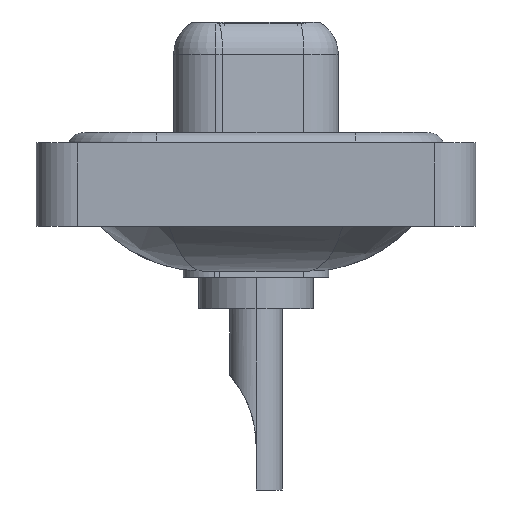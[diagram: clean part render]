
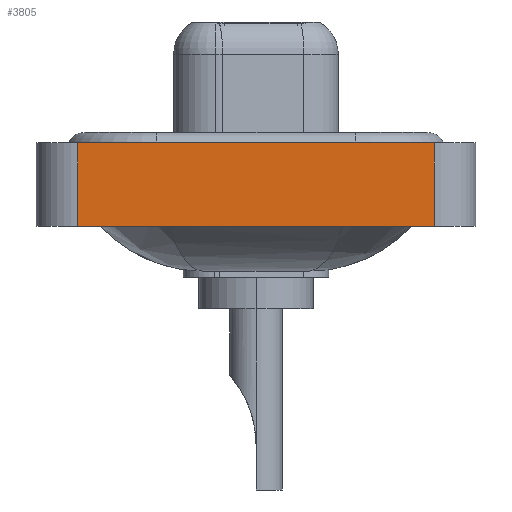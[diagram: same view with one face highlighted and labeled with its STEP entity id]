
A CAD part, left-side view. The second image highlights one B-rep face of the part: STEP entity #3805.
In plain terms, the highlighted planar face has unit normal (-1, 0, 0).
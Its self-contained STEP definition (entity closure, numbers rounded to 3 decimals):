
#897 = ORIENTED_EDGE ( 'NONE', *, *, #14200, .T. ) ;
#1288 = CARTESIAN_POINT ( 'NONE',  ( -7.25, -8.55, -3.6 ) ) ;
#1683 = PLANE ( 'NONE',  #7517 ) ;
#2058 = VECTOR ( 'NONE', #10575, 1000. ) ;
#2520 = CARTESIAN_POINT ( 'NONE',  ( -7.25, -8.55, -3.6 ) ) ;
#2913 = FACE_OUTER_BOUND ( 'NONE', #6104, .T. ) ;
#2992 = DIRECTION ( 'NONE',  ( 0., 0., 1. ) ) ;
#3805 = ADVANCED_FACE ( 'NONE', ( #2913 ), #1683, .T. ) ;
#3864 = EDGE_CURVE ( 'NONE', #12638, #15703, #9419, .T. ) ;
#4318 = ORIENTED_EDGE ( 'NONE', *, *, #7551, .F. ) ;
#4462 = CARTESIAN_POINT ( 'NONE',  ( -7.25, -8.55, -3.6 ) ) ;
#4849 = VECTOR ( 'NONE', #16111, 1000. ) ;
#5597 = DIRECTION ( 'NONE',  ( -1., 0., 0. ) ) ;
#5711 = ORIENTED_EDGE ( 'NONE', *, *, #15212, .F. ) ;
#6010 = CARTESIAN_POINT ( 'NONE',  ( -7.25, 8.55, -3.6 ) ) ;
#6104 = EDGE_LOOP ( 'NONE', ( #14749, #5711, #4318, #897 ) ) ;
#6641 = LINE ( 'NONE', #10410, #11677 ) ;
#7107 = DIRECTION ( 'NONE',  ( 0., -1., 0. ) ) ;
#7247 = VERTEX_POINT ( 'NONE', #6010 ) ;
#7310 = VERTEX_POINT ( 'NONE', #12069 ) ;
#7517 = AXIS2_PLACEMENT_3D ( 'NONE', #4462, #5597, #13421 ) ;
#7551 = EDGE_CURVE ( 'NONE', #7247, #7310, #6641, .T. ) ;
#7723 = CARTESIAN_POINT ( 'NONE',  ( -7.25, -8.55, 0.4 ) ) ;
#8190 = CARTESIAN_POINT ( 'NONE',  ( -7.25, -8.55, -3.6 ) ) ;
#9419 = LINE ( 'NONE', #8190, #2058 ) ;
#9643 = CARTESIAN_POINT ( 'NONE',  ( -7.25, -8.55, 0.4 ) ) ;
#10004 = LINE ( 'NONE', #1288, #4849 ) ;
#10410 = CARTESIAN_POINT ( 'NONE',  ( -7.25, 8.55, -3.6 ) ) ;
#10575 = DIRECTION ( 'NONE',  ( 0., 0., 1. ) ) ;
#11111 = LINE ( 'NONE', #9643, #12195 ) ;
#11677 = VECTOR ( 'NONE', #2992, 1000. ) ;
#12069 = CARTESIAN_POINT ( 'NONE',  ( -7.25, 8.55, 0.4 ) ) ;
#12195 = VECTOR ( 'NONE', #7107, 1000. ) ;
#12638 = VERTEX_POINT ( 'NONE', #2520 ) ;
#13421 = DIRECTION ( 'NONE',  ( 0., 0., 1. ) ) ;
#14200 = EDGE_CURVE ( 'NONE', #7247, #12638, #10004, .T. ) ;
#14749 = ORIENTED_EDGE ( 'NONE', *, *, #3864, .T. ) ;
#15212 = EDGE_CURVE ( 'NONE', #7310, #15703, #11111, .T. ) ;
#15703 = VERTEX_POINT ( 'NONE', #7723 ) ;
#16111 = DIRECTION ( 'NONE',  ( 0., -1., 0. ) ) ;
